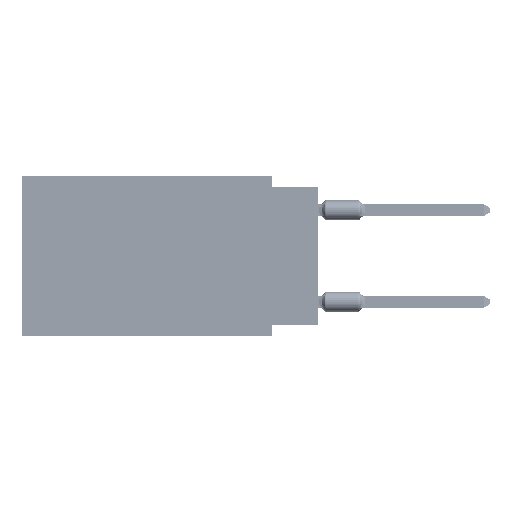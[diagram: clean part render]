
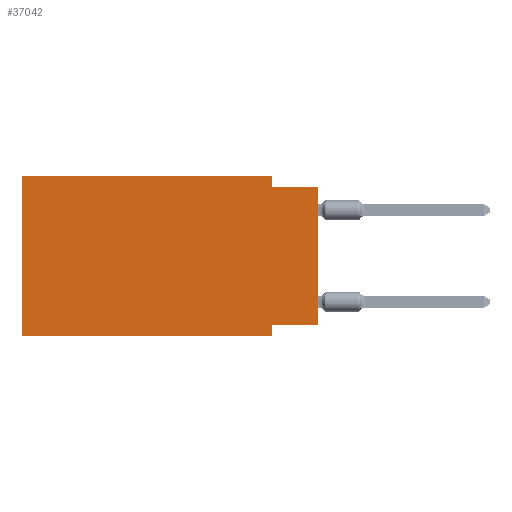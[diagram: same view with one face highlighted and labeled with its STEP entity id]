
A CAD part, left-side view. The second image highlights one B-rep face of the part: STEP entity #37042.
In plain terms, the highlighted planar face has unit normal (-1, 0, 0).
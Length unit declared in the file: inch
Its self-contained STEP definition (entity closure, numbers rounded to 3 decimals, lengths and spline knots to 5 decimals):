
#2668 = CARTESIAN_POINT ( 'NONE',  ( 0., 0., -0.325 ) ) ;
#5266 = LINE ( 'NONE', #101710, #76340 ) ;
#6240 = VECTOR ( 'NONE', #74720, 39.37008 ) ;
#7578 = VECTOR ( 'NONE', #28983, 39.37008 ) ;
#9916 = DIRECTION ( 'NONE',  ( 0., 0., -1. ) ) ;
#13742 = DIRECTION ( 'NONE',  ( 0., -1., 0. ) ) ;
#14225 = DIRECTION ( 'NONE',  ( 0., 0., -1. ) ) ;
#14832 = LINE ( 'NONE', #79455, #66402 ) ;
#16900 = DIRECTION ( 'NONE',  ( 0., -1., 0. ) ) ;
#17239 = ORIENTED_EDGE ( 'NONE', *, *, #102154, .F. ) ;
#17267 = ORIENTED_EDGE ( 'NONE', *, *, #29148, .F. ) ;
#17358 = CARTESIAN_POINT ( 'NONE',  ( 0., 0.1, -0.35 ) ) ;
#17802 = EDGE_CURVE ( 'NONE', #23775, #92473, #5266, .T. ) ;
#23775 = VERTEX_POINT ( 'NONE', #73321 ) ;
#25191 = EDGE_CURVE ( 'NONE', #34009, #92473, #87046, .T. ) ;
#26349 = DIRECTION ( 'NONE',  ( 0., -1., 0. ) ) ;
#26951 = FACE_OUTER_BOUND ( 'NONE', #32675, .T. ) ;
#28983 = DIRECTION ( 'NONE',  ( 0., 0., -1. ) ) ;
#29148 = EDGE_CURVE ( 'NONE', #43744, #54772, #74543, .T. ) ;
#31825 = ORIENTED_EDGE ( 'NONE', *, *, #39555, .T. ) ;
#32675 = EDGE_LOOP ( 'NONE', ( #52130, #35094, #85352, #75433, #88813, #31825, #17267, #17239 ) ) ;
#34009 = VERTEX_POINT ( 'NONE', #86633 ) ;
#35094 = ORIENTED_EDGE ( 'NONE', *, *, #17802, .F. ) ;
#37042 = ADVANCED_FACE ( 'NONE', ( #26951 ), #59249, .F. ) ;
#38635 = VECTOR ( 'NONE', #96055, 39.37008 ) ;
#39555 = EDGE_CURVE ( 'NONE', #41302, #54772, #14832, .T. ) ;
#40265 = VERTEX_POINT ( 'NONE', #60147 ) ;
#41302 = VERTEX_POINT ( 'NONE', #90936 ) ;
#43744 = VERTEX_POINT ( 'NONE', #46360 ) ;
#46360 = CARTESIAN_POINT ( 'NONE',  ( 0., 0.1, -0.325 ) ) ;
#47459 = AXIS2_PLACEMENT_3D ( 'NONE', #91589, #51332, #14225 ) ;
#48108 = CARTESIAN_POINT ( 'NONE',  ( 0., 0., -0.025 ) ) ;
#48911 = CARTESIAN_POINT ( 'NONE',  ( 0., 0.1, 0. ) ) ;
#51332 = DIRECTION ( 'NONE',  ( 1., 0., 0. ) ) ;
#52130 = ORIENTED_EDGE ( 'NONE', *, *, #25191, .T. ) ;
#52468 = CARTESIAN_POINT ( 'NONE',  ( 0., 0.645, 0. ) ) ;
#54711 = VERTEX_POINT ( 'NONE', #48911 ) ;
#54772 = VERTEX_POINT ( 'NONE', #64787 ) ;
#59249 = PLANE ( 'NONE',  #47459 ) ;
#59894 = EDGE_CURVE ( 'NONE', #41302, #40265, #69936, .T. ) ;
#60147 = CARTESIAN_POINT ( 'NONE',  ( 0., 0.645, 0. ) ) ;
#60900 = LINE ( 'NONE', #2668, #6240 ) ;
#64787 = CARTESIAN_POINT ( 'NONE',  ( 0., 0.1, -0.35 ) ) ;
#66402 = VECTOR ( 'NONE', #16900, 39.37008 ) ;
#66603 = LINE ( 'NONE', #98948, #88805 ) ;
#68357 = DIRECTION ( 'NONE',  ( 0., 0., 1. ) ) ;
#68712 = LINE ( 'NONE', #101052, #7578 ) ;
#69936 = LINE ( 'NONE', #52468, #98119 ) ;
#73321 = CARTESIAN_POINT ( 'NONE',  ( 0., 0.1, -0.025 ) ) ;
#74543 = LINE ( 'NONE', #17358, #86596 ) ;
#74720 = DIRECTION ( 'NONE',  ( 0., 1., 0. ) ) ;
#75433 = ORIENTED_EDGE ( 'NONE', *, *, #75676, .F. ) ;
#75676 = EDGE_CURVE ( 'NONE', #40265, #54711, #66603, .T. ) ;
#75833 = EDGE_CURVE ( 'NONE', #54711, #23775, #68712, .T. ) ;
#76340 = VECTOR ( 'NONE', #13742, 39.37008 ) ;
#79455 = CARTESIAN_POINT ( 'NONE',  ( 0., 0.645, -0.35 ) ) ;
#85352 = ORIENTED_EDGE ( 'NONE', *, *, #75833, .F. ) ;
#86596 = VECTOR ( 'NONE', #9916, 39.37008 ) ;
#86633 = CARTESIAN_POINT ( 'NONE',  ( 0., 0., -0.325 ) ) ;
#87046 = LINE ( 'NONE', #88603, #38635 ) ;
#88603 = CARTESIAN_POINT ( 'NONE',  ( 0., 0., 0. ) ) ;
#88805 = VECTOR ( 'NONE', #26349, 39.37008 ) ;
#88813 = ORIENTED_EDGE ( 'NONE', *, *, #59894, .F. ) ;
#90936 = CARTESIAN_POINT ( 'NONE',  ( 0., 0.645, -0.35 ) ) ;
#91589 = CARTESIAN_POINT ( 'NONE',  ( 0., 0.645, 0. ) ) ;
#92473 = VERTEX_POINT ( 'NONE', #48108 ) ;
#96055 = DIRECTION ( 'NONE',  ( 0., 0., 1. ) ) ;
#98119 = VECTOR ( 'NONE', #68357, 39.37008 ) ;
#98948 = CARTESIAN_POINT ( 'NONE',  ( 0., 0.645, 0. ) ) ;
#101052 = CARTESIAN_POINT ( 'NONE',  ( 0., 0.1, 0. ) ) ;
#101710 = CARTESIAN_POINT ( 'NONE',  ( 0., 0., -0.025 ) ) ;
#102154 = EDGE_CURVE ( 'NONE', #34009, #43744, #60900, .T. ) ;
